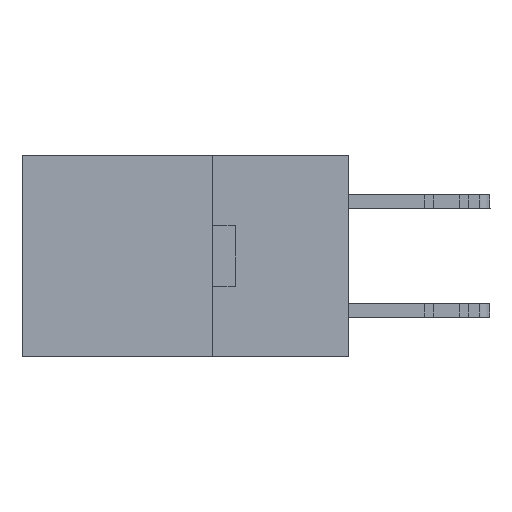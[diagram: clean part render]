
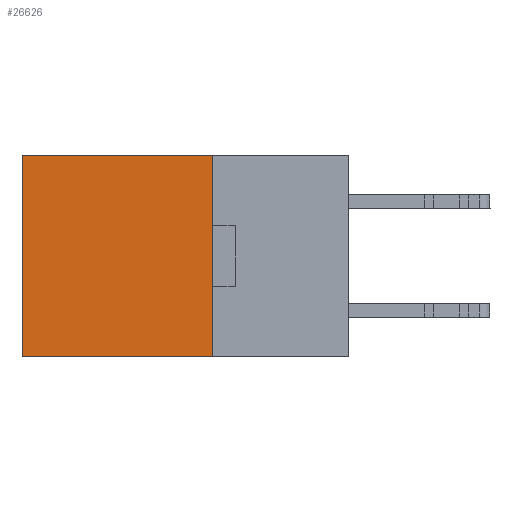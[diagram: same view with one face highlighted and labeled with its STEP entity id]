
A CAD part, left-side view. The second image highlights one B-rep face of the part: STEP entity #26626.
In plain terms, the highlighted planar face has unit normal (-1, 0, 0).
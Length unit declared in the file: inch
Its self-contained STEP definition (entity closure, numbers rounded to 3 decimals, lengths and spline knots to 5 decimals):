
#25 = VECTOR ( 'NONE', #2164, 39.37008 ) ;
#591 = VECTOR ( 'NONE', #5848, 39.37008 ) ;
#1168 = PLANE ( 'NONE',  #1966 ) ;
#1966 = AXIS2_PLACEMENT_3D ( 'NONE', #7753, #22977, #9952 ) ;
#2164 = DIRECTION ( 'NONE',  ( 0., 0., -1. ) ) ;
#3669 = VERTEX_POINT ( 'NONE', #22346 ) ;
#4306 = VECTOR ( 'NONE', #15602, 39.37008 ) ;
#4605 = CARTESIAN_POINT ( 'NONE',  ( 0.2615, 0.25, 0. ) ) ;
#5171 = ORIENTED_EDGE ( 'NONE', *, *, #24939, .F. ) ;
#5848 = DIRECTION ( 'NONE',  ( 0., 1., 0. ) ) ;
#6545 = LINE ( 'NONE', #8653, #25 ) ;
#6696 = EDGE_CURVE ( 'NONE', #10952, #9184, #16610, .T. ) ;
#6803 = CARTESIAN_POINT ( 'NONE',  ( 0.2615, 0.6, -0.37 ) ) ;
#7753 = CARTESIAN_POINT ( 'NONE',  ( 0.2615, 0.25, -0.37 ) ) ;
#8653 = CARTESIAN_POINT ( 'NONE',  ( 0.2615, 0.25, -0.37 ) ) ;
#8961 = ORIENTED_EDGE ( 'NONE', *, *, #16027, .F. ) ;
#9184 = VERTEX_POINT ( 'NONE', #26958 ) ;
#9952 = DIRECTION ( 'NONE',  ( 0., 0., -1. ) ) ;
#10185 = LINE ( 'NONE', #19871, #21094 ) ;
#10803 = EDGE_LOOP ( 'NONE', ( #23711, #8961, #5171, #22777 ) ) ;
#10952 = VERTEX_POINT ( 'NONE', #22047 ) ;
#15602 = DIRECTION ( 'NONE',  ( 0., 0., -1. ) ) ;
#16027 = EDGE_CURVE ( 'NONE', #3669, #9184, #23780, .T. ) ;
#16354 = EDGE_CURVE ( 'NONE', #18301, #10952, #10185, .T. ) ;
#16610 = LINE ( 'NONE', #6803, #4306 ) ;
#16760 = CARTESIAN_POINT ( 'NONE',  ( 0.2615, 0.25, -0.37 ) ) ;
#18301 = VERTEX_POINT ( 'NONE', #4605 ) ;
#19871 = CARTESIAN_POINT ( 'NONE',  ( 0.2615, 0.25, 0. ) ) ;
#21094 = VECTOR ( 'NONE', #24214, 39.37008 ) ;
#22047 = CARTESIAN_POINT ( 'NONE',  ( 0.2615, 0.6, 0. ) ) ;
#22346 = CARTESIAN_POINT ( 'NONE',  ( 0.2615, 0.25, -0.37 ) ) ;
#22777 = ORIENTED_EDGE ( 'NONE', *, *, #16354, .T. ) ;
#22977 = DIRECTION ( 'NONE',  ( 1., 0., 0. ) ) ;
#23711 = ORIENTED_EDGE ( 'NONE', *, *, #6696, .T. ) ;
#23780 = LINE ( 'NONE', #16760, #591 ) ;
#23793 = FACE_OUTER_BOUND ( 'NONE', #10803, .T. ) ;
#24214 = DIRECTION ( 'NONE',  ( 0., 1., 0. ) ) ;
#24939 = EDGE_CURVE ( 'NONE', #18301, #3669, #6545, .T. ) ;
#26626 = ADVANCED_FACE ( 'NONE', ( #23793 ), #1168, .F. ) ;
#26958 = CARTESIAN_POINT ( 'NONE',  ( 0.2615, 0.6, -0.37 ) ) ;
